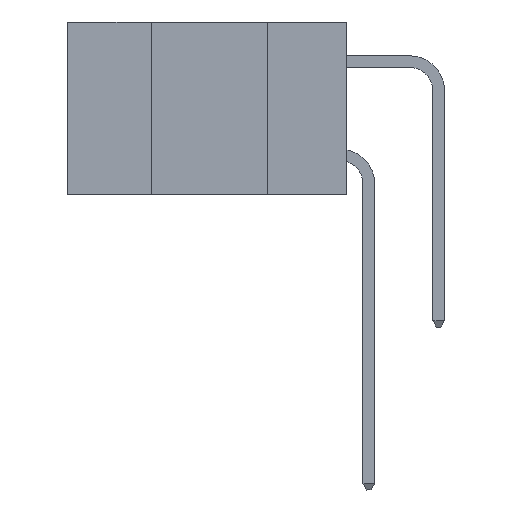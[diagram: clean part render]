
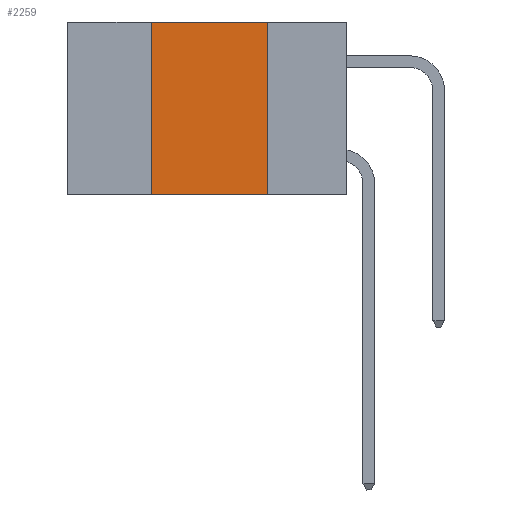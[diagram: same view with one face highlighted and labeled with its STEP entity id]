
A CAD part, left-side view. The second image highlights one B-rep face of the part: STEP entity #2259.
In plain terms, the highlighted planar face has unit normal (-1, 0, 0).
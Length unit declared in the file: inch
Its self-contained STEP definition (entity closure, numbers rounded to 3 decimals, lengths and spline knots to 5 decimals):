
#1405 = ORIENTED_EDGE ( 'NONE', *, *, #12557, .T. ) ;
#1851 = FACE_OUTER_BOUND ( 'NONE', #15787, .T. ) ;
#1913 = VERTEX_POINT ( 'NONE', #6039 ) ;
#2259 = ADVANCED_FACE ( 'NONE', ( #1851 ), #22034, .F. ) ;
#4317 = VECTOR ( 'NONE', #22617, 39.37008 ) ;
#4355 = ORIENTED_EDGE ( 'NONE', *, *, #16126, .F. ) ;
#5523 = CARTESIAN_POINT ( 'NONE',  ( 0., 0.42, 0. ) ) ;
#6039 = CARTESIAN_POINT ( 'NONE',  ( 0., 0.42, -0.37 ) ) ;
#6193 = CARTESIAN_POINT ( 'NONE',  ( 0., 0.17, 0. ) ) ;
#7156 = CARTESIAN_POINT ( 'NONE',  ( 0., 0.6, -0.37 ) ) ;
#7711 = LINE ( 'NONE', #7156, #16656 ) ;
#8552 = AXIS2_PLACEMENT_3D ( 'NONE', #21867, #10646, #10567 ) ;
#8988 = DIRECTION ( 'NONE',  ( 0., -1., 0. ) ) ;
#9597 = VECTOR ( 'NONE', #17816, 39.37008 ) ;
#10567 = DIRECTION ( 'NONE',  ( 0., 0., -1. ) ) ;
#10646 = DIRECTION ( 'NONE',  ( 1., 0., 0. ) ) ;
#12228 = EDGE_CURVE ( 'NONE', #20705, #19236, #14476, .T. ) ;
#12557 = EDGE_CURVE ( 'NONE', #1913, #18677, #7711, .T. ) ;
#12714 = ORIENTED_EDGE ( 'NONE', *, *, #15370, .F. ) ;
#12780 = DIRECTION ( 'NONE',  ( 0., 0., 1. ) ) ;
#13933 = CARTESIAN_POINT ( 'NONE',  ( 0., 0.42, 0. ) ) ;
#14230 = CARTESIAN_POINT ( 'NONE',  ( 0., 0.17, 0. ) ) ;
#14358 = LINE ( 'NONE', #14230, #9597 ) ;
#14476 = LINE ( 'NONE', #20806, #4317 ) ;
#15370 = EDGE_CURVE ( 'NONE', #19236, #18677, #14358, .T. ) ;
#15787 = EDGE_LOOP ( 'NONE', ( #12714, #21375, #4355, #1405 ) ) ;
#16126 = EDGE_CURVE ( 'NONE', #1913, #20705, #22850, .T. ) ;
#16656 = VECTOR ( 'NONE', #8988, 39.37008 ) ;
#17816 = DIRECTION ( 'NONE',  ( 0., 0., -1. ) ) ;
#17948 = VECTOR ( 'NONE', #12780, 39.37008 ) ;
#18677 = VERTEX_POINT ( 'NONE', #22686 ) ;
#19236 = VERTEX_POINT ( 'NONE', #6193 ) ;
#20705 = VERTEX_POINT ( 'NONE', #13933 ) ;
#20806 = CARTESIAN_POINT ( 'NONE',  ( 0., 0.6, 0. ) ) ;
#21375 = ORIENTED_EDGE ( 'NONE', *, *, #12228, .F. ) ;
#21867 = CARTESIAN_POINT ( 'NONE',  ( 0., 0.6, 0. ) ) ;
#22034 = PLANE ( 'NONE',  #8552 ) ;
#22617 = DIRECTION ( 'NONE',  ( 0., -1., 0. ) ) ;
#22686 = CARTESIAN_POINT ( 'NONE',  ( 0., 0.17, -0.37 ) ) ;
#22850 = LINE ( 'NONE', #5523, #17948 ) ;
